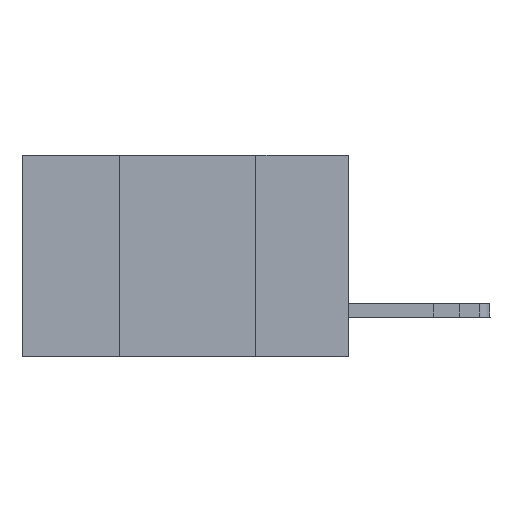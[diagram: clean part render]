
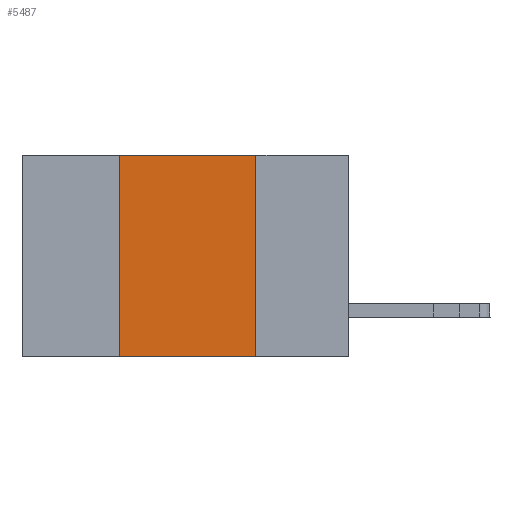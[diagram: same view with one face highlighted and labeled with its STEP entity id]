
A CAD part, left-side view. The second image highlights one B-rep face of the part: STEP entity #5487.
In plain terms, the highlighted planar face has unit normal (-1, 0, 0).
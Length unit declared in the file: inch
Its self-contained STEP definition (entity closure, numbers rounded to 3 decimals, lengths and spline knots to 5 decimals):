
#206 = EDGE_CURVE ( 'NONE', #16470, #17650, #9811, .T. ) ;
#1810 = AXIS2_PLACEMENT_3D ( 'NONE', #1969, #9432, #11057 ) ;
#1969 = CARTESIAN_POINT ( 'NONE',  ( 0., 0.6, 0. ) ) ;
#2916 = DIRECTION ( 'NONE',  ( 0., 0., -1. ) ) ;
#3089 = EDGE_CURVE ( 'NONE', #6948, #17650, #16327, .T. ) ;
#3400 = EDGE_CURVE ( 'NONE', #21438, #6948, #21042, .T. ) ;
#4053 = ORIENTED_EDGE ( 'NONE', *, *, #206, .T. ) ;
#5487 = ADVANCED_FACE ( 'NONE', ( #22599 ), #5584, .F. ) ;
#5584 = PLANE ( 'NONE',  #1810 ) ;
#5714 = CARTESIAN_POINT ( 'NONE',  ( 0., 0.42, 0. ) ) ;
#6948 = VERTEX_POINT ( 'NONE', #17984 ) ;
#9432 = DIRECTION ( 'NONE',  ( 1., 0., 0. ) ) ;
#9811 = LINE ( 'NONE', #16897, #18664 ) ;
#10909 = ORIENTED_EDGE ( 'NONE', *, *, #3400, .F. ) ;
#11057 = DIRECTION ( 'NONE',  ( 0., 0., -1. ) ) ;
#11069 = VECTOR ( 'NONE', #20769, 39.37008 ) ;
#13185 = CARTESIAN_POINT ( 'NONE',  ( 0., 0.42, 0. ) ) ;
#13330 = CARTESIAN_POINT ( 'NONE',  ( 0., 0.6, 0. ) ) ;
#15631 = VECTOR ( 'NONE', #18685, 39.37008 ) ;
#16327 = LINE ( 'NONE', #18322, #20685 ) ;
#16470 = VERTEX_POINT ( 'NONE', #17730 ) ;
#16897 = CARTESIAN_POINT ( 'NONE',  ( 0., 0.6, -0.37 ) ) ;
#17300 = LINE ( 'NONE', #13185, #11069 ) ;
#17392 = DIRECTION ( 'NONE',  ( 0., -1., 0. ) ) ;
#17650 = VERTEX_POINT ( 'NONE', #22729 ) ;
#17730 = CARTESIAN_POINT ( 'NONE',  ( 0., 0.42, -0.37 ) ) ;
#17984 = CARTESIAN_POINT ( 'NONE',  ( 0., 0.17, 0. ) ) ;
#18322 = CARTESIAN_POINT ( 'NONE',  ( 0., 0.17, 0. ) ) ;
#18664 = VECTOR ( 'NONE', #17392, 39.37008 ) ;
#18685 = DIRECTION ( 'NONE',  ( 0., -1., 0. ) ) ;
#19555 = EDGE_LOOP ( 'NONE', ( #24212, #10909, #23898, #4053 ) ) ;
#19856 = EDGE_CURVE ( 'NONE', #16470, #21438, #17300, .T. ) ;
#20685 = VECTOR ( 'NONE', #2916, 39.37008 ) ;
#20769 = DIRECTION ( 'NONE',  ( 0., 0., 1. ) ) ;
#21042 = LINE ( 'NONE', #13330, #15631 ) ;
#21438 = VERTEX_POINT ( 'NONE', #5714 ) ;
#22599 = FACE_OUTER_BOUND ( 'NONE', #19555, .T. ) ;
#22729 = CARTESIAN_POINT ( 'NONE',  ( 0., 0.17, -0.37 ) ) ;
#23898 = ORIENTED_EDGE ( 'NONE', *, *, #19856, .F. ) ;
#24212 = ORIENTED_EDGE ( 'NONE', *, *, #3089, .F. ) ;
